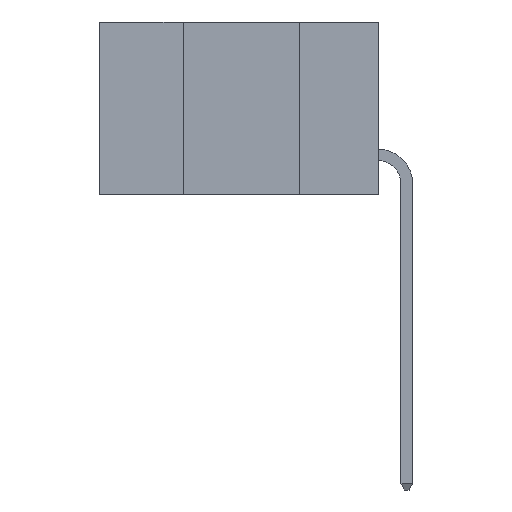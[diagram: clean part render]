
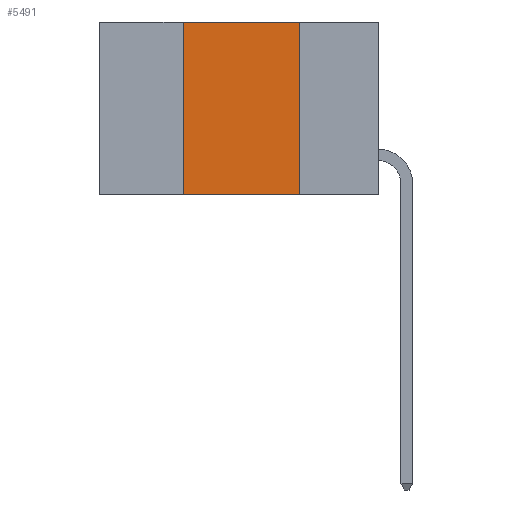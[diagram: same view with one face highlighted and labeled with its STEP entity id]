
A CAD part, left-side view. The second image highlights one B-rep face of the part: STEP entity #5491.
In plain terms, the highlighted planar face has unit normal (-1, 0, 0).
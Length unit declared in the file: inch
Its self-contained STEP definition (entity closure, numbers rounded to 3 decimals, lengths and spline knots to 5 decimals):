
#208 = LINE ( 'NONE', #12115, #3083 ) ;
#773 = CARTESIAN_POINT ( 'NONE',  ( 0., 0.42, -0.37 ) ) ;
#1702 = VERTEX_POINT ( 'NONE', #10145 ) ;
#1864 = PLANE ( 'NONE',  #9948 ) ;
#2020 = DIRECTION ( 'NONE',  ( 0., 0., -1. ) ) ;
#2359 = EDGE_CURVE ( 'NONE', #5135, #4311, #208, .T. ) ;
#2762 = LINE ( 'NONE', #4057, #10212 ) ;
#2938 = DIRECTION ( 'NONE',  ( 0., 0., -1. ) ) ;
#3064 = EDGE_CURVE ( 'NONE', #5135, #8009, #2762, .T. ) ;
#3075 = CARTESIAN_POINT ( 'NONE',  ( 0., 0.17, -0.37 ) ) ;
#3083 = VECTOR ( 'NONE', #12145, 39.37008 ) ;
#3295 = DIRECTION ( 'NONE',  ( 0., 0., 1. ) ) ;
#3718 = CARTESIAN_POINT ( 'NONE',  ( 0., 0.6, 0. ) ) ;
#4057 = CARTESIAN_POINT ( 'NONE',  ( 0., 0.42, -0.37 ) ) ;
#4182 = CARTESIAN_POINT ( 'NONE',  ( 0., 0.17, -0.37 ) ) ;
#4311 = VERTEX_POINT ( 'NONE', #4182 ) ;
#4981 = CARTESIAN_POINT ( 'NONE',  ( 0., 0.6, 0. ) ) ;
#5135 = VERTEX_POINT ( 'NONE', #773 ) ;
#5491 = ADVANCED_FACE ( 'NONE', ( #11278 ), #1864, .F. ) ;
#5828 = ORIENTED_EDGE ( 'NONE', *, *, #10109, .F. ) ;
#6086 = VECTOR ( 'NONE', #2020, 39.37008 ) ;
#6396 = LINE ( 'NONE', #3075, #6086 ) ;
#6713 = VECTOR ( 'NONE', #9759, 39.37008 ) ;
#8009 = VERTEX_POINT ( 'NONE', #11044 ) ;
#8485 = EDGE_LOOP ( 'NONE', ( #5828, #10142, #8861, #9289 ) ) ;
#8861 = ORIENTED_EDGE ( 'NONE', *, *, #3064, .F. ) ;
#9054 = DIRECTION ( 'NONE',  ( 1., 0., 0. ) ) ;
#9289 = ORIENTED_EDGE ( 'NONE', *, *, #2359, .T. ) ;
#9759 = DIRECTION ( 'NONE',  ( 0., -1., 0. ) ) ;
#9948 = AXIS2_PLACEMENT_3D ( 'NONE', #4981, #9054, #2938 ) ;
#10109 = EDGE_CURVE ( 'NONE', #1702, #4311, #6396, .T. ) ;
#10142 = ORIENTED_EDGE ( 'NONE', *, *, #10501, .F. ) ;
#10145 = CARTESIAN_POINT ( 'NONE',  ( 0., 0.17, 0. ) ) ;
#10212 = VECTOR ( 'NONE', #3295, 39.37008 ) ;
#10501 = EDGE_CURVE ( 'NONE', #8009, #1702, #11917, .T. ) ;
#11044 = CARTESIAN_POINT ( 'NONE',  ( 0., 0.42, 0. ) ) ;
#11278 = FACE_OUTER_BOUND ( 'NONE', #8485, .T. ) ;
#11917 = LINE ( 'NONE', #3718, #6713 ) ;
#12115 = CARTESIAN_POINT ( 'NONE',  ( 0., 0.6, -0.37 ) ) ;
#12145 = DIRECTION ( 'NONE',  ( 0., -1., 0. ) ) ;
